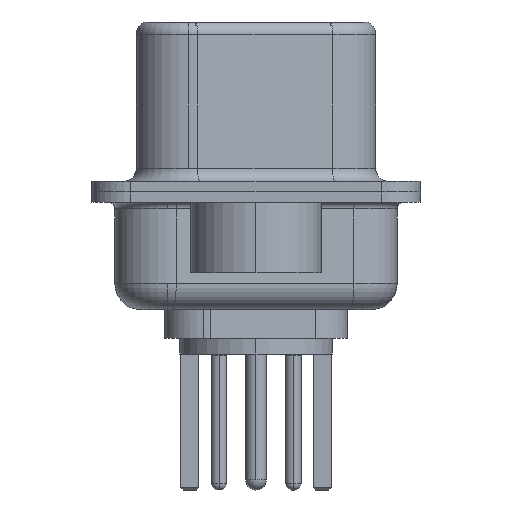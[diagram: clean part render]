
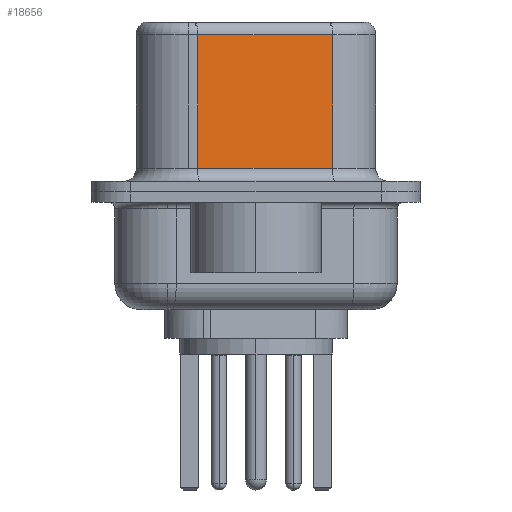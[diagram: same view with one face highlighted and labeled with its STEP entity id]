
A CAD part, left-side view. The second image highlights one B-rep face of the part: STEP entity #18656.
In plain terms, the highlighted planar face has unit normal (-0.985, -0.174, 0).
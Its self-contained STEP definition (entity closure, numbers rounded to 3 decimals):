
#1172 = DIRECTION ( 'NONE',  ( -0.174, 0.985, 0. ) ) ;
#1343 = ORIENTED_EDGE ( 'NONE', *, *, #10066, .T. ) ;
#1625 = CARTESIAN_POINT ( 'NONE',  ( 4.58, -2.927, 0.9 ) ) ;
#3456 = EDGE_LOOP ( 'NONE', ( #13243, #15891, #11696, #1343 ) ) ;
#3564 = VERTEX_POINT ( 'NONE', #4023 ) ;
#3845 = LINE ( 'NONE', #4011, #21203 ) ;
#4011 = CARTESIAN_POINT ( 'NONE',  ( 3.67, 2.233, 6.52 ) ) ;
#4023 = CARTESIAN_POINT ( 'NONE',  ( 4.58, -2.927, 6.02 ) ) ;
#4876 = LINE ( 'NONE', #9207, #17719 ) ;
#5580 = LINE ( 'NONE', #20716, #13897 ) ;
#6422 = CARTESIAN_POINT ( 'NONE',  ( 4.58, -2.927, 6.02 ) ) ;
#6927 = VERTEX_POINT ( 'NONE', #12153 ) ;
#7820 = EDGE_CURVE ( 'NONE', #3564, #20763, #4876, .T. ) ;
#9107 = FACE_OUTER_BOUND ( 'NONE', #3456, .T. ) ;
#9207 = CARTESIAN_POINT ( 'NONE',  ( 4.58, -2.927, 6.52 ) ) ;
#10066 = EDGE_CURVE ( 'NONE', #6927, #20763, #5580, .T. ) ;
#10597 = DIRECTION ( 'NONE',  ( 0.174, -0.985, 0. ) ) ;
#10779 = VERTEX_POINT ( 'NONE', #18987 ) ;
#11148 = DIRECTION ( 'NONE',  ( 0.985, 0.174, 0. ) ) ;
#11589 = AXIS2_PLACEMENT_3D ( 'NONE', #21239, #11148, #1172 ) ;
#11696 = ORIENTED_EDGE ( 'NONE', *, *, #13034, .T. ) ;
#12083 = EDGE_CURVE ( 'NONE', #3564, #10779, #16126, .T. ) ;
#12153 = CARTESIAN_POINT ( 'NONE',  ( 3.67, 2.233, 0.9 ) ) ;
#12206 = VECTOR ( 'NONE', #18170, 1000. ) ;
#13034 = EDGE_CURVE ( 'NONE', #10779, #6927, #3845, .T. ) ;
#13243 = ORIENTED_EDGE ( 'NONE', *, *, #7820, .F. ) ;
#13897 = VECTOR ( 'NONE', #10597, 1000. ) ;
#15891 = ORIENTED_EDGE ( 'NONE', *, *, #12083, .T. ) ;
#15995 = DIRECTION ( 'NONE',  ( 0., 0., -1. ) ) ;
#16126 = LINE ( 'NONE', #6422, #12206 ) ;
#17719 = VECTOR ( 'NONE', #15995, 1000. ) ;
#18170 = DIRECTION ( 'NONE',  ( -0.174, 0.985, 0. ) ) ;
#18656 = ADVANCED_FACE ( 'NONE', ( #9107 ), #21318, .F. ) ;
#18987 = CARTESIAN_POINT ( 'NONE',  ( 3.67, 2.233, 6.02 ) ) ;
#20716 = CARTESIAN_POINT ( 'NONE',  ( 4.58, -2.927, 0.9 ) ) ;
#20763 = VERTEX_POINT ( 'NONE', #1625 ) ;
#20823 = DIRECTION ( 'NONE',  ( 0., 0., -1. ) ) ;
#21203 = VECTOR ( 'NONE', #20823, 1000. ) ;
#21239 = CARTESIAN_POINT ( 'NONE',  ( 4.58, -2.927, 6.52 ) ) ;
#21318 = PLANE ( 'NONE',  #11589 ) ;
